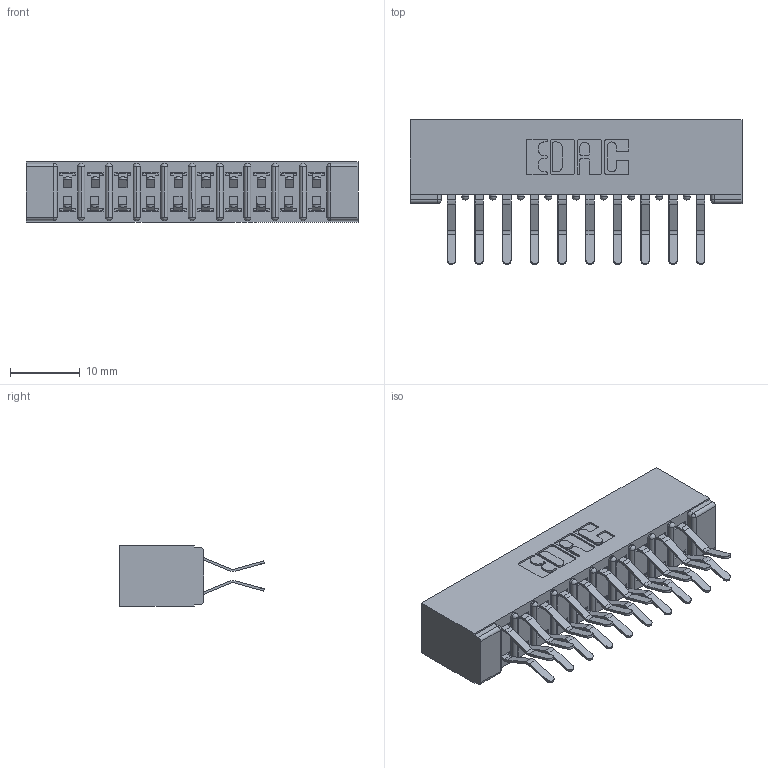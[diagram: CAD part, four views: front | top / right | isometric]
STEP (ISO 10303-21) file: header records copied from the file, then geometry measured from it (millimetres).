
FILE_DESCRIPTION (( 'STEP AP203' ), '1' );
FILE_NAME ('357-020-560-201.STEP', '2019-09-17T20:54:55', ( '' ), ( '' ), 'SwSTEP 2.0', 'SolidWorks 2016', '' );
FILE_SCHEMA (( 'CONFIG_CONTROL_DESIGN' ));
Length unit declared in the file: inch
Products named in the file (3): 357-020-560-201; 307 Part_No Mounting Lugs; 307-290-001_560
Assembly tree (21 placements, depth 2):
  357-020-560-201
    307 Part_No Mounting Lugs
    307-290-001_560  x20
Bounding box: 47.5 x 20.73 x 8.71 mm (x, y, z)
Volume: 3366.3 mm3; surface area: 5941.9 mm2
Topology: 21 solids, 21 shells, 1121 faces, 3139 edges, 2034 vertices
Faces by surface type: plane 726, cylinder 373, sphere 22
Entity records: 12664 total; most frequent: CARTESIAN_POINT 2078, ORIENTED_EDGE 2054, DIRECTION 2049, EDGE_CURVE 1027, VECTOR 775, LINE 775, VERTEX_POINT 666, AXIS2_PLACEMENT_3D 637
